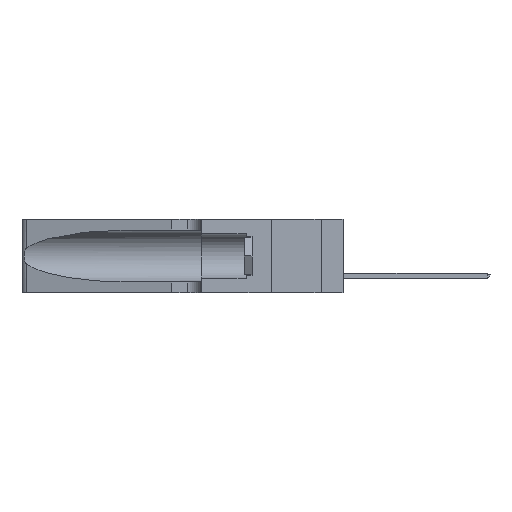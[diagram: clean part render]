
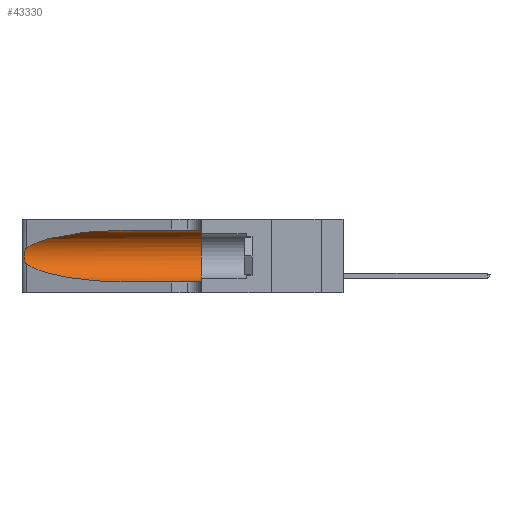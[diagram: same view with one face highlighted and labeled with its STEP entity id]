
A CAD part, left-side view. The second image highlights one B-rep face of the part: STEP entity #43330.
In plain terms, the highlighted cylindrical face has radius 3.308 mm (diameter 6.617 mm), a partial arc.
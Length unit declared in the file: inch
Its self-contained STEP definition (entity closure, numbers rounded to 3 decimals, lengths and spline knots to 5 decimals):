
#871 = CARTESIAN_POINT ( 'NONE',  ( 0.1305, 0.35, 0.185 ) ) ;
#2693 = CARTESIAN_POINT ( 'NONE',  ( 0.25555, 1.22994, 0.2215 ) ) ;
#3562 = LINE ( 'NONE', #41197, #23190 ) ;
#4268 = DIRECTION ( 'NONE',  ( 0., 0., -1. ) ) ;
#4272 = CARTESIAN_POINT ( 'NONE',  ( 0.1305, 0.72297, 0.05475 ) ) ;
#4400 = CARTESIAN_POINT ( 'NONE',  ( 0.1305, 0.72297, 0.05475 ) ) ;
#4533 = ORIENTED_EDGE ( 'NONE', *, *, #15116, .T. ) ;
#7023 = CARTESIAN_POINT ( 'NONE',  ( 0.25856, 1.23593, 0.16098 ) ) ;
#10074 = AXIS2_PLACEMENT_3D ( 'NONE', #871, #13044, #42153 ) ;
#10244 = CARTESIAN_POINT ( 'NONE',  ( 0.25487, 1.22718, 0.14631 ) ) ;
#10343 = ORIENTED_EDGE ( 'NONE', *, *, #25850, .T. ) ;
#10617 =( BOUNDED_CURVE ( )  B_SPLINE_CURVE ( 3, ( #18032, #13995, #29184, #21293 ),
 .UNSPECIFIED., .F., .T. ) 
 B_SPLINE_CURVE_WITH_KNOTS ( ( 4, 4 ),
 ( 1.5708, 2.84003 ),
 .UNSPECIFIED. ) 
 CURVE ( )  GEOMETRIC_REPRESENTATION_ITEM ( )  RATIONAL_B_SPLINE_CURVE ( ( 1., 0.87, 0.87, 1. ) ) 
 REPRESENTATION_ITEM ( '' )  );
#11522 = CARTESIAN_POINT ( 'NONE',  ( 0.25487, 1.22718, 0.14631 ) ) ;
#12739 = EDGE_CURVE ( 'NONE', #38270, #30839, #3562, .T. ) ;
#12800 = VECTOR ( 'NONE', #21848, 39.37008 ) ;
#13044 = DIRECTION ( 'NONE',  ( 0., 1., 0. ) ) ;
#13074 = VERTEX_POINT ( 'NONE', #42004 ) ;
#13149 = CARTESIAN_POINT ( 'NONE',  ( 0.26018, 1.23835, 0.19895 ) ) ;
#13995 = CARTESIAN_POINT ( 'NONE',  ( 0.18966, 0.96281, 0.31525 ) ) ;
#14109 = CARTESIAN_POINT ( 'NONE',  ( 0.26017, 1.23833, 0.17102 ) ) ;
#15116 = EDGE_CURVE ( 'NONE', #28587, #32104, #10617, .T. ) ;
#17682 = CARTESIAN_POINT ( 'NONE',  ( 0.25555, 1.22993, 0.14849 ) ) ;
#18032 = CARTESIAN_POINT ( 'NONE',  ( 0.1305, 0.72297, 0.31525 ) ) ;
#19277 = CARTESIAN_POINT ( 'NONE',  ( 0.2373, 1.15595, 0.08982 ) ) ;
#19466 = ORIENTED_EDGE ( 'NONE', *, *, #35527, .T. ) ;
#19518 = EDGE_CURVE ( 'NONE', #13074, #30839, #34873, .T. ) ;
#20278 = CYLINDRICAL_SURFACE ( 'NONE', #38595, 0.13025 ) ;
#21253 = CARTESIAN_POINT ( 'NONE',  ( 0.25789, 1.23486, 0.15765 ) ) ;
#21293 = CARTESIAN_POINT ( 'NONE',  ( 0.25487, 1.22718, 0.22369 ) ) ;
#21591 = ORIENTED_EDGE ( 'NONE', *, *, #19518, .F. ) ;
#21848 = DIRECTION ( 'NONE',  ( 0., -1., 0. ) ) ;
#22526 = CARTESIAN_POINT ( 'NONE',  ( 0.18966, 0.96281, 0.05475 ) ) ;
#22925 = DIRECTION ( 'NONE',  ( 0., -1., 0. ) ) ;
#23190 = VECTOR ( 'NONE', #22925, 39.37008 ) ;
#23804 = EDGE_LOOP ( 'NONE', ( #4533, #19466, #10343, #33337, #21591, #24123 ) ) ;
#24123 = ORIENTED_EDGE ( 'NONE', *, *, #38909, .F. ) ;
#24487 = CARTESIAN_POINT ( 'NONE',  ( 0.25854, 1.2359, 0.20912 ) ) ;
#25129 = CARTESIAN_POINT ( 'NONE',  ( 0.26075, 1.23896, 0.178 ) ) ;
#25850 = EDGE_CURVE ( 'NONE', #44336, #38270, #26749, .T. ) ;
#26406 = DIRECTION ( 'NONE',  ( 0., -1., 0. ) ) ;
#26749 =( BOUNDED_CURVE ( )  B_SPLINE_CURVE ( 3, ( #11522, #19277, #22526, #4400 ),
 .UNSPECIFIED., .F., .F. ) 
 B_SPLINE_CURVE_WITH_KNOTS ( ( 4, 4 ),
 ( 3.44316, 4.71239 ),
 .UNSPECIFIED. ) 
 CURVE ( )  GEOMETRIC_REPRESENTATION_ITEM ( )  RATIONAL_B_SPLINE_CURVE ( ( 1., 0.87, 0.87, 1. ) ) 
 REPRESENTATION_ITEM ( '' )  );
#26915 = CARTESIAN_POINT ( 'NONE',  ( 0.25487, 1.22718, 0.14631 ) ) ;
#26951 = CARTESIAN_POINT ( 'NONE',  ( 0.25487, 1.22718, 0.22369 ) ) ;
#27883 = CARTESIAN_POINT ( 'NONE',  ( 0.25787, 1.23484, 0.2124 ) ) ;
#28587 = VERTEX_POINT ( 'NONE', #44034 ) ;
#29184 = CARTESIAN_POINT ( 'NONE',  ( 0.2373, 1.15595, 0.28018 ) ) ;
#29228 = CARTESIAN_POINT ( 'NONE',  ( 0.1305, 0.35, 0.05475 ) ) ;
#30839 = VERTEX_POINT ( 'NONE', #29228 ) ;
#32104 = VERTEX_POINT ( 'NONE', #26951 ) ;
#32230 = B_SPLINE_CURVE_WITH_KNOTS ( 'NONE', 3,
 ( #46809, #2693, #35915, #27883, #24487, #13149, #36235, #25129, #14109, #7023, #21253, #32809, #17682, #10244 ),
 .UNSPECIFIED., .F., .F.,
 ( 4, 2, 2, 2, 2, 2, 4 ),
 ( 0., 0.00027, 0.00053, 0.00107, 0.0016, 0.00187, 0.00214 ),
 .UNSPECIFIED. ) ;
#32809 = CARTESIAN_POINT ( 'NONE',  ( 0.25639, 1.23186, 0.15144 ) ) ;
#33337 = ORIENTED_EDGE ( 'NONE', *, *, #12739, .T. ) ;
#34873 = CIRCLE ( 'NONE', #10074, 0.13025 ) ;
#35527 = EDGE_CURVE ( 'NONE', #32104, #44336, #32230, .T. ) ;
#35915 = CARTESIAN_POINT ( 'NONE',  ( 0.25639, 1.23184, 0.21858 ) ) ;
#36235 = CARTESIAN_POINT ( 'NONE',  ( 0.26075, 1.23896, 0.19203 ) ) ;
#38270 = VERTEX_POINT ( 'NONE', #4272 ) ;
#38595 = AXIS2_PLACEMENT_3D ( 'NONE', #45648, #26406, #4268 ) ;
#38909 = EDGE_CURVE ( 'NONE', #28587, #13074, #44617, .T. ) ;
#41197 = CARTESIAN_POINT ( 'NONE',  ( 0.1305, 1.61858, 0.05475 ) ) ;
#42004 = CARTESIAN_POINT ( 'NONE',  ( 0.1305, 0.35, 0.31525 ) ) ;
#42153 = DIRECTION ( 'NONE',  ( 0., 0., 1. ) ) ;
#42855 = FACE_OUTER_BOUND ( 'NONE', #23804, .T. ) ;
#43330 = ADVANCED_FACE ( 'NONE', ( #42855 ), #20278, .F. ) ;
#44034 = CARTESIAN_POINT ( 'NONE',  ( 0.1305, 0.72297, 0.31525 ) ) ;
#44336 = VERTEX_POINT ( 'NONE', #26915 ) ;
#44617 = LINE ( 'NONE', #47898, #12800 ) ;
#45648 = CARTESIAN_POINT ( 'NONE',  ( 0.1305, 1.61858, 0.185 ) ) ;
#46809 = CARTESIAN_POINT ( 'NONE',  ( 0.25487, 1.22718, 0.22369 ) ) ;
#47898 = CARTESIAN_POINT ( 'NONE',  ( 0.1305, 1.61858, 0.31525 ) ) ;
